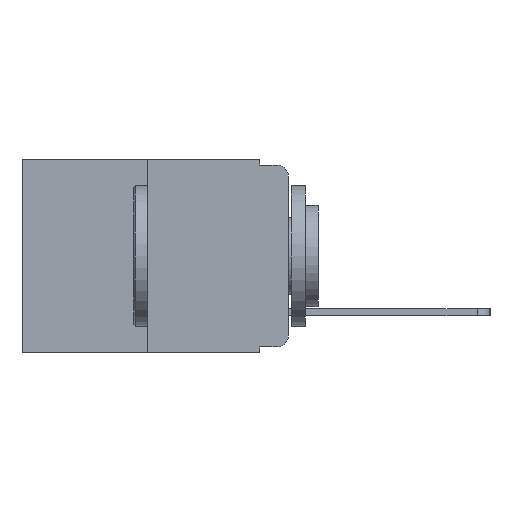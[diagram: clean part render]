
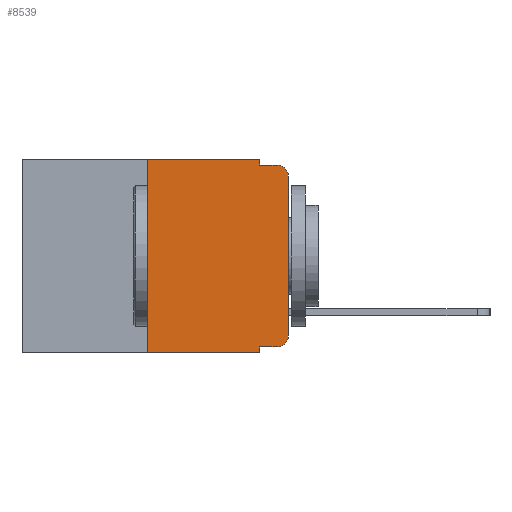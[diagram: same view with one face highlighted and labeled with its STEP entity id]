
A CAD part, left-side view. The second image highlights one B-rep face of the part: STEP entity #8539.
In plain terms, the highlighted planar face has unit normal (-1, 0, 0).
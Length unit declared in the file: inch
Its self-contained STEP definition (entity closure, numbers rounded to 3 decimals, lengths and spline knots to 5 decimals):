
#44 = ORIENTED_EDGE ( 'NONE', *, *, #2240, .F. ) ;
#629 = CARTESIAN_POINT ( 'NONE',  ( 0., 0.051, -0.01 ) ) ;
#661 = VERTEX_POINT ( 'NONE', #8097 ) ;
#706 = DIRECTION ( 'NONE',  ( -1., 0., 0. ) ) ;
#778 = EDGE_CURVE ( 'NONE', #3013, #661, #16517, .T. ) ;
#837 = AXIS2_PLACEMENT_3D ( 'NONE', #9442, #706, #10887 ) ;
#1072 = CARTESIAN_POINT ( 'NONE',  ( 0., 0.02, -0.01 ) ) ;
#1255 = CARTESIAN_POINT ( 'NONE',  ( 0., 0.473, 0. ) ) ;
#1274 = CARTESIAN_POINT ( 'NONE',  ( 0., 0.25, 0. ) ) ;
#1473 = VERTEX_POINT ( 'NONE', #3568 ) ;
#1544 = VECTOR ( 'NONE', #8907, 39.37008 ) ;
#1554 = VERTEX_POINT ( 'NONE', #5486 ) ;
#1864 = VECTOR ( 'NONE', #8041, 39.37008 ) ;
#1986 = LINE ( 'NONE', #1274, #1544 ) ;
#2027 = ORIENTED_EDGE ( 'NONE', *, *, #6630, .F. ) ;
#2240 = EDGE_CURVE ( 'NONE', #5305, #7866, #17115, .T. ) ;
#2284 = VECTOR ( 'NONE', #3212, 39.37008 ) ;
#2742 = DIRECTION ( 'NONE',  ( 1., 0., 0. ) ) ;
#2755 = EDGE_CURVE ( 'NONE', #3422, #3013, #7337, .T. ) ;
#2783 = VECTOR ( 'NONE', #6553, 39.37008 ) ;
#2971 = VECTOR ( 'NONE', #4213, 39.37008 ) ;
#2983 = EDGE_CURVE ( 'NONE', #1473, #1554, #7101, .T. ) ;
#3013 = VERTEX_POINT ( 'NONE', #14288 ) ;
#3124 = CARTESIAN_POINT ( 'NONE',  ( 0., 0.051, -0.01 ) ) ;
#3212 = DIRECTION ( 'NONE',  ( 0., -1., 0. ) ) ;
#3422 = VERTEX_POINT ( 'NONE', #12480 ) ;
#3568 = CARTESIAN_POINT ( 'NONE',  ( 0., 0.25, -0.343 ) ) ;
#3672 = EDGE_CURVE ( 'NONE', #3422, #1554, #5921, .T. ) ;
#3707 = AXIS2_PLACEMENT_3D ( 'NONE', #1255, #2742, #12857 ) ;
#3905 = ORIENTED_EDGE ( 'NONE', *, *, #3672, .F. ) ;
#4088 = VERTEX_POINT ( 'NONE', #7619 ) ;
#4202 = ORIENTED_EDGE ( 'NONE', *, *, #2755, .T. ) ;
#4213 = DIRECTION ( 'NONE',  ( 0., 0., -1. ) ) ;
#4640 = EDGE_CURVE ( 'NONE', #1473, #5305, #1986, .T. ) ;
#5305 = VERTEX_POINT ( 'NONE', #18371 ) ;
#5481 = ORIENTED_EDGE ( 'NONE', *, *, #4640, .F. ) ;
#5486 = CARTESIAN_POINT ( 'NONE',  ( 0., 0.051, -0.343 ) ) ;
#5671 = EDGE_CURVE ( 'NONE', #7866, #13326, #7446, .T. ) ;
#5690 = ORIENTED_EDGE ( 'NONE', *, *, #5671, .F. ) ;
#5921 = LINE ( 'NONE', #7048, #2971 ) ;
#6154 = LINE ( 'NONE', #629, #2284 ) ;
#6553 = DIRECTION ( 'NONE',  ( 0., -1., 0. ) ) ;
#6630 = EDGE_CURVE ( 'NONE', #13326, #7286, #6154, .T. ) ;
#7048 = CARTESIAN_POINT ( 'NONE',  ( 0., 0.051, 0. ) ) ;
#7101 = LINE ( 'NONE', #16481, #2783 ) ;
#7239 = DIRECTION ( 'NONE',  ( 0., 0., 1. ) ) ;
#7286 = VERTEX_POINT ( 'NONE', #1072 ) ;
#7337 = LINE ( 'NONE', #11041, #11192 ) ;
#7446 = LINE ( 'NONE', #14027, #18266 ) ;
#7494 = VECTOR ( 'NONE', #7239, 39.37008 ) ;
#7605 = EDGE_CURVE ( 'NONE', #4088, #7286, #13348, .T. ) ;
#7619 = CARTESIAN_POINT ( 'NONE',  ( 0., 0., -0.03 ) ) ;
#7839 = ORIENTED_EDGE ( 'NONE', *, *, #8624, .T. ) ;
#7857 = ORIENTED_EDGE ( 'NONE', *, *, #7605, .T. ) ;
#7866 = VERTEX_POINT ( 'NONE', #18381 ) ;
#8041 = DIRECTION ( 'NONE',  ( 0., -1., 0. ) ) ;
#8097 = CARTESIAN_POINT ( 'NONE',  ( 0., 0., -0.313 ) ) ;
#8312 = ORIENTED_EDGE ( 'NONE', *, *, #778, .T. ) ;
#8539 = ADVANCED_FACE ( 'NONE', ( #12692 ), #11438, .F. ) ;
#8624 = EDGE_CURVE ( 'NONE', #661, #4088, #15086, .T. ) ;
#8718 = EDGE_LOOP ( 'NONE', ( #7839, #7857, #2027, #5690, #44, #5481, #13923, #3905, #4202, #8312 ) ) ;
#8907 = DIRECTION ( 'NONE',  ( 0., 0., 1. ) ) ;
#9442 = CARTESIAN_POINT ( 'NONE',  ( 0., 0.02, -0.03 ) ) ;
#9546 = AXIS2_PLACEMENT_3D ( 'NONE', #15851, #15816, #10276 ) ;
#10276 = DIRECTION ( 'NONE',  ( 0., 0., -1. ) ) ;
#10887 = DIRECTION ( 'NONE',  ( 0., 0., -1. ) ) ;
#11041 = CARTESIAN_POINT ( 'NONE',  ( 0., 0.051, -0.333 ) ) ;
#11192 = VECTOR ( 'NONE', #17221, 39.37008 ) ;
#11438 = PLANE ( 'NONE',  #3707 ) ;
#11563 = CARTESIAN_POINT ( 'NONE',  ( 0., 0., 0. ) ) ;
#12480 = CARTESIAN_POINT ( 'NONE',  ( 0., 0.051, -0.333 ) ) ;
#12692 = FACE_OUTER_BOUND ( 'NONE', #8718, .T. ) ;
#12857 = DIRECTION ( 'NONE',  ( 0., 0., -1. ) ) ;
#13284 = CARTESIAN_POINT ( 'NONE',  ( 0., 0.473, 0. ) ) ;
#13326 = VERTEX_POINT ( 'NONE', #3124 ) ;
#13348 = CIRCLE ( 'NONE', #837, 0.02 ) ;
#13893 = DIRECTION ( 'NONE',  ( 0., 0., -1. ) ) ;
#13923 = ORIENTED_EDGE ( 'NONE', *, *, #2983, .T. ) ;
#14027 = CARTESIAN_POINT ( 'NONE',  ( 0., 0.051, 0. ) ) ;
#14288 = CARTESIAN_POINT ( 'NONE',  ( 0., 0.02, -0.333 ) ) ;
#15086 = LINE ( 'NONE', #11563, #7494 ) ;
#15816 = DIRECTION ( 'NONE',  ( -1., 0., 0. ) ) ;
#15851 = CARTESIAN_POINT ( 'NONE',  ( 0., 0.02, -0.313 ) ) ;
#16481 = CARTESIAN_POINT ( 'NONE',  ( 0., 0.473, -0.343 ) ) ;
#16517 = CIRCLE ( 'NONE', #9546, 0.02 ) ;
#17115 = LINE ( 'NONE', #13284, #1864 ) ;
#17221 = DIRECTION ( 'NONE',  ( 0., -1., 0. ) ) ;
#18266 = VECTOR ( 'NONE', #13893, 39.37008 ) ;
#18371 = CARTESIAN_POINT ( 'NONE',  ( 0., 0.25, 0. ) ) ;
#18381 = CARTESIAN_POINT ( 'NONE',  ( 0., 0.051, 0. ) ) ;
